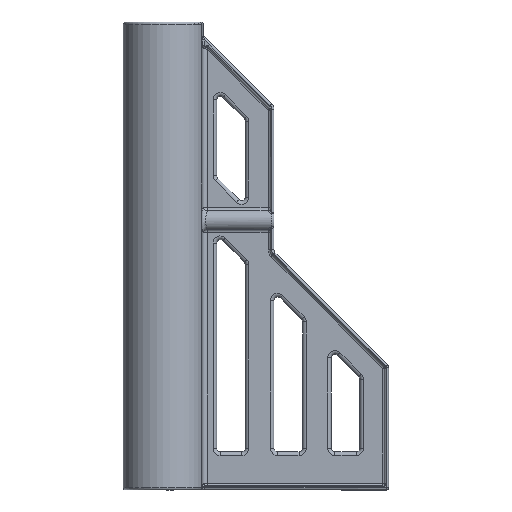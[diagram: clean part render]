
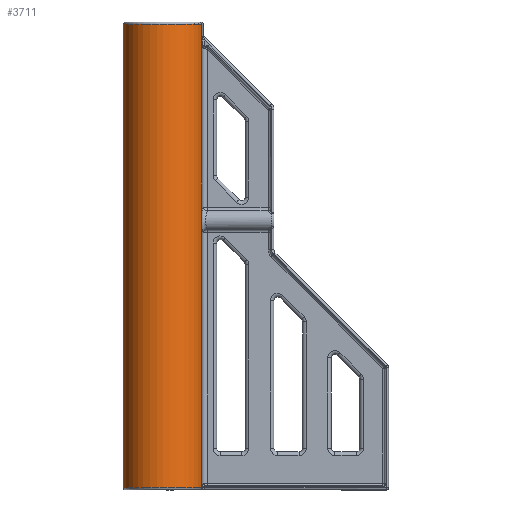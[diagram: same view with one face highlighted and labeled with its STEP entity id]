
A CAD part, left-side view. The second image highlights one B-rep face of the part: STEP entity #3711.
In plain terms, the highlighted cylindrical face has radius 17.833 mm (diameter 35.667 mm), a partial arc.
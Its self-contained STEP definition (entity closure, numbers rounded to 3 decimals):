
#336=CYLINDRICAL_SURFACE('',#4166,17.833);
#531=FACE_OUTER_BOUND('',#778,.T.);
#778=EDGE_LOOP('',(#3259,#3260,#3261,#3262,#3263,#3264,#3265));
#906=LINE('',#6477,#1106);
#920=LINE('',#6821,#1120);
#921=LINE('',#6822,#1121);
#962=LINE('',#7621,#1162);
#963=LINE('',#7624,#1163);
#1106=VECTOR('',#4538,10.);
#1120=VECTOR('',#4626,10.);
#1121=VECTOR('',#4627,10.);
#1162=VECTOR('',#4858,10.);
#1163=VECTOR('',#4861,10.);
#1253=CIRCLE('',#3827,17.833);
#1465=CIRCLE('',#4167,17.833);
#1554=VERTEX_POINT('',#5757);
#1557=VERTEX_POINT('',#5776);
#1631=VERTEX_POINT('',#6476);
#1663=VERTEX_POINT('',#6814);
#1664=VERTEX_POINT('',#6820);
#1758=VERTEX_POINT('',#7620);
#1759=VERTEX_POINT('',#7622);
#1901=EDGE_CURVE('',#1557,#1554,#1253,.T.);
#2004=EDGE_CURVE('',#1631,#1554,#906,.T.);
#2056=EDGE_CURVE('',#1663,#1664,#920,.T.);
#2057=EDGE_CURVE('',#1664,#1557,#921,.T.);
#2193=EDGE_CURVE('',#1758,#1631,#962,.T.);
#2195=EDGE_CURVE('',#1759,#1663,#963,.T.);
#2339=EDGE_CURVE('',#1758,#1759,#1465,.T.);
#3259=ORIENTED_EDGE('',*,*,#1901,.F.);
#3260=ORIENTED_EDGE('',*,*,#2057,.F.);
#3261=ORIENTED_EDGE('',*,*,#2056,.F.);
#3262=ORIENTED_EDGE('',*,*,#2195,.F.);
#3263=ORIENTED_EDGE('',*,*,#2339,.F.);
#3264=ORIENTED_EDGE('',*,*,#2193,.T.);
#3265=ORIENTED_EDGE('',*,*,#2004,.T.);
#3711=ADVANCED_FACE('',(#531),#336,.T.);
#3827=AXIS2_PLACEMENT_3D('',#5789,#4368,#4369);
#4166=AXIS2_PLACEMENT_3D('',#7939,#5207,#5208);
#4167=AXIS2_PLACEMENT_3D('',#7940,#5209,#5210);
#4368=DIRECTION('center_axis',(0.,0.,
-1.));
#4369=DIRECTION('ref_axis',(0.,1.,0.));
#4538=DIRECTION('',(0.,0.,-1.));
#4626=DIRECTION('',(0.,0.,-1.));
#4627=DIRECTION('',(0.,0.,-1.));
#4858=DIRECTION('',(0.,0.,-1.));
#4861=DIRECTION('',(0.,0.,-1.));
#5207=DIRECTION('center_axis',(0.,0.,-1.));
#5208=DIRECTION('ref_axis',(0.,1.,0.));
#5209=DIRECTION('center_axis',(0.,0.,1.));
#5210=DIRECTION('ref_axis',(0.,1.,0.));
#5757=CARTESIAN_POINT('',(6.227,-22.401,-3.185));
#5776=CARTESIAN_POINT('',(-6.227,-22.401,-3.185));
#5789=CARTESIAN_POINT('Origin',(0.,-5.69,
-3.185));
#6476=CARTESIAN_POINT('',(6.227,-22.401,115.389));
#6477=CARTESIAN_POINT('',(6.227,-22.401,203.2));
#6814=CARTESIAN_POINT('',(-6.227,-22.401,115.389));
#6820=CARTESIAN_POINT('',(-6.227,-22.401,-3.175));
#6821=CARTESIAN_POINT('',(-6.227,-22.401,203.2));
#6822=CARTESIAN_POINT('',(-6.227,-22.401,203.2));
#7620=CARTESIAN_POINT('',(6.227,-22.401,202.2));
#7621=CARTESIAN_POINT('',(6.227,-22.401,203.2));
#7622=CARTESIAN_POINT('',(-6.227,-22.401,202.2));
#7624=CARTESIAN_POINT('',(-6.227,-22.401,203.2));
#7939=CARTESIAN_POINT('Origin',(0.,-5.69,
203.2));
#7940=CARTESIAN_POINT('Origin',(0.,-5.69,
202.2));
